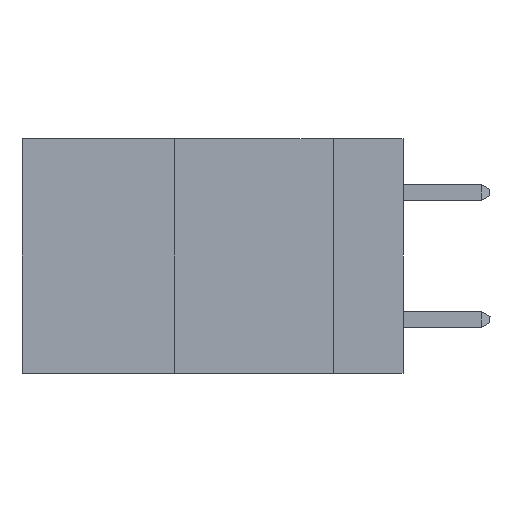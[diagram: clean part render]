
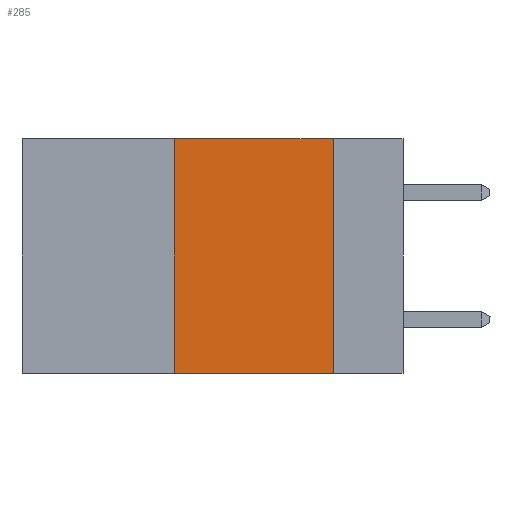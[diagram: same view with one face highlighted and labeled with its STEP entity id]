
A CAD part, left-side view. The second image highlights one B-rep face of the part: STEP entity #285.
In plain terms, the highlighted planar face has unit normal (-1, 0, 0).
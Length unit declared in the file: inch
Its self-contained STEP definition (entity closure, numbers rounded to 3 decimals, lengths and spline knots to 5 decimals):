
#285 = ADVANCED_FACE ( 'NONE', ( #2950 ), #3139, .F. ) ;
#644 = CARTESIAN_POINT ( 'NONE',  ( 0., 0.11, 0. ) ) ;
#934 = DIRECTION ( 'NONE',  ( 0., -1., 0. ) ) ;
#1292 = CARTESIAN_POINT ( 'NONE',  ( 0., 0.6, 0. ) ) ;
#1727 = CARTESIAN_POINT ( 'NONE',  ( 0., 0.6, -0.37 ) ) ;
#2201 = DIRECTION ( 'NONE',  ( 0., -1., 0. ) ) ;
#2685 = EDGE_LOOP ( 'NONE', ( #10700, #6227, #10586, #8237 ) ) ;
#2866 = LINE ( 'NONE', #4582, #4570 ) ;
#2910 = DIRECTION ( 'NONE',  ( 0., 0., -1. ) ) ;
#2950 = FACE_OUTER_BOUND ( 'NONE', #2685, .T. ) ;
#3055 = LINE ( 'NONE', #1292, #4345 ) ;
#3104 = VERTEX_POINT ( 'NONE', #10738 ) ;
#3139 = PLANE ( 'NONE',  #7402 ) ;
#4345 = VECTOR ( 'NONE', #2201, 39.37008 ) ;
#4570 = VECTOR ( 'NONE', #10325, 39.37008 ) ;
#4582 = CARTESIAN_POINT ( 'NONE',  ( 0., 0.36, 0. ) ) ;
#4593 = VERTEX_POINT ( 'NONE', #644 ) ;
#4692 = CARTESIAN_POINT ( 'NONE',  ( 0., 0.11, -0.37 ) ) ;
#5335 = EDGE_CURVE ( 'NONE', #3104, #4593, #3055, .T. ) ;
#5371 = CARTESIAN_POINT ( 'NONE',  ( 0., 0.36, -0.37 ) ) ;
#5945 = DIRECTION ( 'NONE',  ( 0., 0., -1. ) ) ;
#6227 = ORIENTED_EDGE ( 'NONE', *, *, #5335, .F. ) ;
#6862 = CARTESIAN_POINT ( 'NONE',  ( 0., 0.6, 0. ) ) ;
#6889 = EDGE_CURVE ( 'NONE', #7436, #3104, #2866, .T. ) ;
#7174 = VECTOR ( 'NONE', #2910, 39.37008 ) ;
#7402 = AXIS2_PLACEMENT_3D ( 'NONE', #6862, #10601, #5945 ) ;
#7436 = VERTEX_POINT ( 'NONE', #5371 ) ;
#7463 = LINE ( 'NONE', #1727, #9292 ) ;
#7490 = LINE ( 'NONE', #8244, #7174 ) ;
#8237 = ORIENTED_EDGE ( 'NONE', *, *, #11313, .T. ) ;
#8244 = CARTESIAN_POINT ( 'NONE',  ( 0., 0.11, 0. ) ) ;
#9221 = EDGE_CURVE ( 'NONE', #4593, #9223, #7490, .T. ) ;
#9223 = VERTEX_POINT ( 'NONE', #4692 ) ;
#9292 = VECTOR ( 'NONE', #934, 39.37008 ) ;
#10325 = DIRECTION ( 'NONE',  ( 0., 0., 1. ) ) ;
#10586 = ORIENTED_EDGE ( 'NONE', *, *, #6889, .F. ) ;
#10601 = DIRECTION ( 'NONE',  ( 1., 0., 0. ) ) ;
#10700 = ORIENTED_EDGE ( 'NONE', *, *, #9221, .F. ) ;
#10738 = CARTESIAN_POINT ( 'NONE',  ( 0., 0.36, 0. ) ) ;
#11313 = EDGE_CURVE ( 'NONE', #7436, #9223, #7463, .T. ) ;
